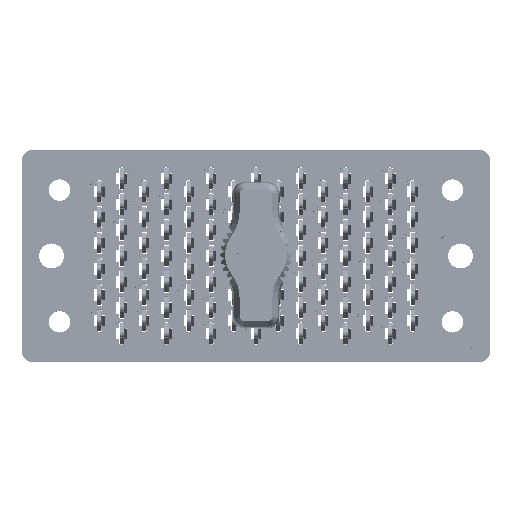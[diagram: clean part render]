
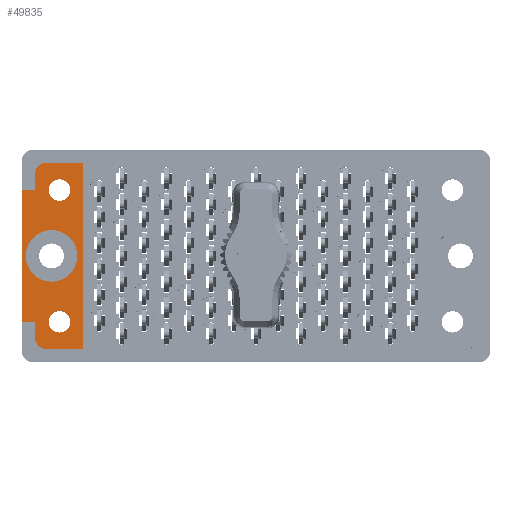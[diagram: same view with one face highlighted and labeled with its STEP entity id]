
A CAD part, top view. The second image highlights one B-rep face of the part: STEP entity #49835.
In plain terms, the highlighted planar face has unit normal (0, 0, 1).
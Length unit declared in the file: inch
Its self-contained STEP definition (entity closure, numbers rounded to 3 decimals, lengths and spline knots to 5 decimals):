
#138 = VECTOR ( 'NONE', #30080, 39.37008 ) ;
#516 = CARTESIAN_POINT ( 'NONE',  ( -1.0785, -0.3825, -0.117 ) ) ;
#683 = LINE ( 'NONE', #21981, #73114 ) ;
#891 = FACE_BOUND ( 'NONE', #60992, .T. ) ;
#1737 = CIRCLE ( 'NONE', #22037, 0.15 ) ;
#2303 = DIRECTION ( 'NONE',  ( 0., 0., 1. ) ) ;
#2623 = DIRECTION ( 'NONE',  ( 0., 0., 1. ) ) ;
#3450 = DIRECTION ( 'NONE',  ( 0., -1., 0. ) ) ;
#3538 = CARTESIAN_POINT ( 'NONE',  ( 0., -0.54, -0.117 ) ) ;
#3975 = FACE_BOUND ( 'NONE', #6710, .T. ) ;
#4118 = EDGE_LOOP ( 'NONE', ( #6747, #51487 ) ) ;
#5054 = VERTEX_POINT ( 'NONE', #44638 ) ;
#5228 = LINE ( 'NONE', #29123, #38908 ) ;
#5979 = AXIS2_PLACEMENT_3D ( 'NONE', #30910, #17645, #11148 ) ;
#5984 = DIRECTION ( 'NONE',  ( 1., 0., 0. ) ) ;
#6176 = DIRECTION ( 'NONE',  ( 1., 0., 0. ) ) ;
#6318 = VERTEX_POINT ( 'NONE', #33812 ) ;
#6534 = DIRECTION ( 'NONE',  ( 0., 0., 1. ) ) ;
#6710 = EDGE_LOOP ( 'NONE', ( #63520, #47086 ) ) ;
#6747 = ORIENTED_EDGE ( 'NONE', *, *, #34264, .F. ) ;
#6803 = EDGE_CURVE ( 'NONE', #31354, #33011, #77570, .T. ) ;
#8177 = DIRECTION ( 'NONE',  ( 0., 0., 1. ) ) ;
#9025 = DIRECTION ( 'NONE',  ( 1., 0., 0. ) ) ;
#9078 = ORIENTED_EDGE ( 'NONE', *, *, #34989, .T. ) ;
#9218 = EDGE_CURVE ( 'NONE', #81091, #9866, #77648, .T. ) ;
#9523 = LINE ( 'NONE', #3538, #138 ) ;
#9866 = VERTEX_POINT ( 'NONE', #516 ) ;
#10400 = CARTESIAN_POINT ( 'NONE',  ( -1.2825, -0.3825, -0.117 ) ) ;
#11148 = DIRECTION ( 'NONE',  ( 1., 0., 0. ) ) ;
#11822 = EDGE_CURVE ( 'NONE', #37377, #5054, #1737, .T. ) ;
#15254 = DIRECTION ( 'NONE',  ( 1., 0., 0. ) ) ;
#15287 = CARTESIAN_POINT ( 'NONE',  ( -1.0785, 0.3825, -0.117 ) ) ;
#15639 = CARTESIAN_POINT ( 'NONE',  ( -1.2035, 0.3825, -0.117 ) ) ;
#16066 = ORIENTED_EDGE ( 'NONE', *, *, #53608, .T. ) ;
#17645 = DIRECTION ( 'NONE',  ( 0., 0., 1. ) ) ;
#21981 = CARTESIAN_POINT ( 'NONE',  ( 0., -0.3825, -0.117 ) ) ;
#22037 = AXIS2_PLACEMENT_3D ( 'NONE', #48171, #2303, #9025 ) ;
#23030 = CARTESIAN_POINT ( 'NONE',  ( -1.141, 0.3825, -0.117 ) ) ;
#23078 = VERTEX_POINT ( 'NONE', #80303 ) ;
#23531 = CARTESIAN_POINT ( 'NONE',  ( -1.0375, 0., -0.117 ) ) ;
#25570 = VERTEX_POINT ( 'NONE', #68002 ) ;
#26897 = LINE ( 'NONE', #68932, #57372 ) ;
#27456 = AXIS2_PLACEMENT_3D ( 'NONE', #82862, #8177, #27962 ) ;
#27902 = LINE ( 'NONE', #38079, #48853 ) ;
#27962 = DIRECTION ( 'NONE',  ( 1., 0., 0. ) ) ;
#28903 = VERTEX_POINT ( 'NONE', #15639 ) ;
#29123 = CARTESIAN_POINT ( 'NONE',  ( -1.359, 0.617, -0.117 ) ) ;
#29345 = LINE ( 'NONE', #57147, #49288 ) ;
#29361 = CARTESIAN_POINT ( 'NONE',  ( -1.359, 0.3825, -0.117 ) ) ;
#29550 = CARTESIAN_POINT ( 'NONE',  ( -1.359, -0.3825, -0.117 ) ) ;
#29621 = DIRECTION ( 'NONE',  ( -1., 0., 0. ) ) ;
#30039 = AXIS2_PLACEMENT_3D ( 'NONE', #36701, #2623, #15254 ) ;
#30080 = DIRECTION ( 'NONE',  ( -1., 0., 0. ) ) ;
#30910 = CARTESIAN_POINT ( 'NONE',  ( -1.141, -0.3825, -0.117 ) ) ;
#31212 = VERTEX_POINT ( 'NONE', #10400 ) ;
#31354 = VERTEX_POINT ( 'NONE', #74073 ) ;
#31494 = EDGE_CURVE ( 'NONE', #77830, #28903, #49163, .T. ) ;
#32432 = FACE_OUTER_BOUND ( 'NONE', #65745, .T. ) ;
#32615 = EDGE_CURVE ( 'NONE', #31212, #40048, #683, .T. ) ;
#33011 = VERTEX_POINT ( 'NONE', #34499 ) ;
#33499 = CIRCLE ( 'NONE', #45921, 0.062 ) ;
#33812 = CARTESIAN_POINT ( 'NONE',  ( -1.2825, 0.478, -0.117 ) ) ;
#33931 = DIRECTION ( 'NONE',  ( 0., 0., 1. ) ) ;
#34264 = EDGE_CURVE ( 'NONE', #28903, #77830, #61489, .T. ) ;
#34499 = CARTESIAN_POINT ( 'NONE',  ( -1.2205, 0.54, -0.117 ) ) ;
#34989 = EDGE_CURVE ( 'NONE', #33011, #6318, #86603, .T. ) ;
#35165 = ORIENTED_EDGE ( 'NONE', *, *, #38726, .F. ) ;
#35955 = CIRCLE ( 'NONE', #55282, 0.15 ) ;
#36074 = ORIENTED_EDGE ( 'NONE', *, *, #9218, .F. ) ;
#36274 = LINE ( 'NONE', #56974, #52074 ) ;
#36447 = EDGE_CURVE ( 'NONE', #9866, #81091, #56941, .T. ) ;
#36701 = CARTESIAN_POINT ( 'NONE',  ( -1.359, -0.617, -0.117 ) ) ;
#36771 = DIRECTION ( 'NONE',  ( 0., 0., 1. ) ) ;
#37377 = VERTEX_POINT ( 'NONE', #23531 ) ;
#38079 = CARTESIAN_POINT ( 'NONE',  ( -1.2825, 0., -0.117 ) ) ;
#38726 = EDGE_CURVE ( 'NONE', #41409, #23078, #9523, .T. ) ;
#38908 = VECTOR ( 'NONE', #3450, 39.37008 ) ;
#40048 = VERTEX_POINT ( 'NONE', #29550 ) ;
#41409 = VERTEX_POINT ( 'NONE', #63633 ) ;
#42237 = DIRECTION ( 'NONE',  ( 0., -1., 0. ) ) ;
#43466 = DIRECTION ( 'NONE',  ( -1., 0., 0. ) ) ;
#44638 = CARTESIAN_POINT ( 'NONE',  ( -1.3375, 0., -0.117 ) ) ;
#44762 = VERTEX_POINT ( 'NONE', #29361 ) ;
#45750 = ORIENTED_EDGE ( 'NONE', *, *, #36447, .F. ) ;
#45921 = AXIS2_PLACEMENT_3D ( 'NONE', #59989, #66986, #6176 ) ;
#47086 = ORIENTED_EDGE ( 'NONE', *, *, #47627, .F. ) ;
#47627 = EDGE_CURVE ( 'NONE', #5054, #37377, #35955, .T. ) ;
#48171 = CARTESIAN_POINT ( 'NONE',  ( -1.1875, 0., -0.117 ) ) ;
#48564 = EDGE_CURVE ( 'NONE', #44762, #40048, #5228, .T. ) ;
#48853 = VECTOR ( 'NONE', #77437, 39.37008 ) ;
#49163 = CIRCLE ( 'NONE', #58168, 0.0625 ) ;
#49288 = VECTOR ( 'NONE', #57448, 39.37008 ) ;
#49360 = PLANE ( 'NONE',  #30039 ) ;
#49722 = DIRECTION ( 'NONE',  ( 1., 0., 0. ) ) ;
#49835 = ADVANCED_FACE ( 'NONE', ( #891, #52436, #3975, #32432 ), #49360, .T. ) ;
#50755 = EDGE_CURVE ( 'NONE', #25570, #44762, #36274, .T. ) ;
#51487 = ORIENTED_EDGE ( 'NONE', *, *, #31494, .F. ) ;
#51568 = EDGE_CURVE ( 'NONE', #41409, #31354, #29345, .T. ) ;
#52074 = VECTOR ( 'NONE', #43466, 39.37008 ) ;
#52436 = FACE_BOUND ( 'NONE', #4118, .T. ) ;
#53369 = CARTESIAN_POINT ( 'NONE',  ( -1.1875, 0., -0.117 ) ) ;
#53608 = EDGE_CURVE ( 'NONE', #6318, #25570, #26897, .T. ) ;
#53639 = DIRECTION ( 'NONE',  ( 1., 0., 0. ) ) ;
#55282 = AXIS2_PLACEMENT_3D ( 'NONE', #53369, #33931, #5984 ) ;
#56941 = CIRCLE ( 'NONE', #59582, 0.0625 ) ;
#56974 = CARTESIAN_POINT ( 'NONE',  ( 0., 0.3825, -0.117 ) ) ;
#57008 = ORIENTED_EDGE ( 'NONE', *, *, #32615, .F. ) ;
#57147 = CARTESIAN_POINT ( 'NONE',  ( -1.005, 0.617, -0.117 ) ) ;
#57372 = VECTOR ( 'NONE', #42237, 39.37008 ) ;
#57448 = DIRECTION ( 'NONE',  ( 0., 1., 0. ) ) ;
#58168 = AXIS2_PLACEMENT_3D ( 'NONE', #23030, #36771, #49722 ) ;
#58553 = ORIENTED_EDGE ( 'NONE', *, *, #85620, .T. ) ;
#59488 = DIRECTION ( 'NONE',  ( -1., 0., 0. ) ) ;
#59582 = AXIS2_PLACEMENT_3D ( 'NONE', #65295, #72328, #85905 ) ;
#59989 = CARTESIAN_POINT ( 'NONE',  ( -1.2205, -0.478, -0.117 ) ) ;
#60992 = EDGE_LOOP ( 'NONE', ( #36074, #45750 ) ) ;
#61489 = CIRCLE ( 'NONE', #86492, 0.0625 ) ;
#63520 = ORIENTED_EDGE ( 'NONE', *, *, #11822, .F. ) ;
#63633 = CARTESIAN_POINT ( 'NONE',  ( -1.005, -0.54, -0.117 ) ) ;
#65295 = CARTESIAN_POINT ( 'NONE',  ( -1.141, -0.3825, -0.117 ) ) ;
#65745 = EDGE_LOOP ( 'NONE', ( #58553, #70788, #35165, #81769, #76786, #9078, #16066, #68017, #66097, #57008 ) ) ;
#66097 = ORIENTED_EDGE ( 'NONE', *, *, #48564, .T. ) ;
#66986 = DIRECTION ( 'NONE',  ( 0., 0., 1. ) ) ;
#67346 = CARTESIAN_POINT ( 'NONE',  ( -1.141, 0.3825, -0.117 ) ) ;
#68002 = CARTESIAN_POINT ( 'NONE',  ( -1.2825, 0.3825, -0.117 ) ) ;
#68017 = ORIENTED_EDGE ( 'NONE', *, *, #50755, .T. ) ;
#68932 = CARTESIAN_POINT ( 'NONE',  ( -1.2825, 0., -0.117 ) ) ;
#70788 = ORIENTED_EDGE ( 'NONE', *, *, #79628, .T. ) ;
#72328 = DIRECTION ( 'NONE',  ( 0., 0., 1. ) ) ;
#72425 = VERTEX_POINT ( 'NONE', #85569 ) ;
#73114 = VECTOR ( 'NONE', #29621, 39.37008 ) ;
#73508 = CARTESIAN_POINT ( 'NONE',  ( 0., 0.54, -0.117 ) ) ;
#74073 = CARTESIAN_POINT ( 'NONE',  ( -1.005, 0.54, -0.117 ) ) ;
#75234 = CARTESIAN_POINT ( 'NONE',  ( -1.2035, -0.3825, -0.117 ) ) ;
#76556 = VECTOR ( 'NONE', #59488, 39.37008 ) ;
#76786 = ORIENTED_EDGE ( 'NONE', *, *, #6803, .T. ) ;
#77437 = DIRECTION ( 'NONE',  ( 0., -1., 0. ) ) ;
#77570 = LINE ( 'NONE', #73508, #76556 ) ;
#77648 = CIRCLE ( 'NONE', #5979, 0.0625 ) ;
#77830 = VERTEX_POINT ( 'NONE', #15287 ) ;
#79628 = EDGE_CURVE ( 'NONE', #72425, #23078, #33499, .T. ) ;
#80303 = CARTESIAN_POINT ( 'NONE',  ( -1.2205, -0.54, -0.117 ) ) ;
#81091 = VERTEX_POINT ( 'NONE', #75234 ) ;
#81769 = ORIENTED_EDGE ( 'NONE', *, *, #51568, .T. ) ;
#82862 = CARTESIAN_POINT ( 'NONE',  ( -1.2205, 0.478, -0.117 ) ) ;
#85569 = CARTESIAN_POINT ( 'NONE',  ( -1.2825, -0.478, -0.117 ) ) ;
#85620 = EDGE_CURVE ( 'NONE', #31212, #72425, #27902, .T. ) ;
#85905 = DIRECTION ( 'NONE',  ( 1., 0., 0. ) ) ;
#86492 = AXIS2_PLACEMENT_3D ( 'NONE', #67346, #6534, #53639 ) ;
#86603 = CIRCLE ( 'NONE', #27456, 0.062 ) ;
